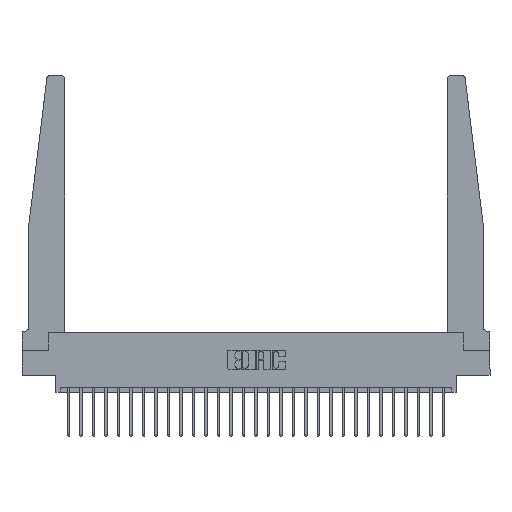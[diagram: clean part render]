
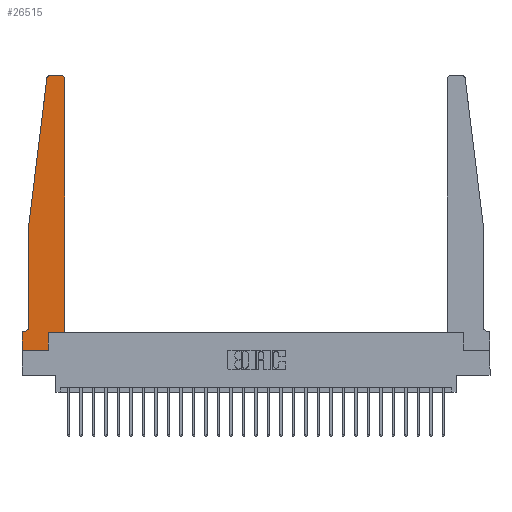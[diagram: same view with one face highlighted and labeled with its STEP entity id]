
A CAD part, top view. The second image highlights one B-rep face of the part: STEP entity #26515.
In plain terms, the highlighted planar face has unit normal (0, 0, 1).
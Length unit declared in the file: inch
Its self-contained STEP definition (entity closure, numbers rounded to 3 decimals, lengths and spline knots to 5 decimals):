
#359 = CARTESIAN_POINT ( 'NONE',  ( 0., 0., 0.37 ) ) ;
#526 = PLANE ( 'NONE',  #13266 ) ;
#586 = VERTEX_POINT ( 'NONE', #23461 ) ;
#639 = DIRECTION ( 'NONE',  ( -1., 0., 0. ) ) ;
#808 = DIRECTION ( 'NONE',  ( 1., 0., 0. ) ) ;
#1301 = LINE ( 'NONE', #24404, #22584 ) ;
#1389 = LINE ( 'NONE', #4986, #22674 ) ;
#1801 = VECTOR ( 'NONE', #2415, 39.37008 ) ;
#1988 = CARTESIAN_POINT ( 'NONE',  ( 0., 0., 0.37 ) ) ;
#2281 = CARTESIAN_POINT ( 'NONE',  ( 0.425, 0.18, 0.37 ) ) ;
#2287 = VECTOR ( 'NONE', #23270, 39.37008 ) ;
#2310 = VERTEX_POINT ( 'NONE', #2281 ) ;
#2415 = DIRECTION ( 'NONE',  ( -1., 0., 0. ) ) ;
#2443 = EDGE_CURVE ( 'NONE', #22834, #11309, #18690, .T. ) ;
#2521 = EDGE_CURVE ( 'NONE', #2310, #586, #22271, .T. ) ;
#2590 = DIRECTION ( 'NONE',  ( 0., 0., 1. ) ) ;
#2798 = EDGE_CURVE ( 'NONE', #4115, #15857, #1301, .T. ) ;
#3279 = CARTESIAN_POINT ( 'NONE',  ( 0.065, 1.25, 0.37 ) ) ;
#4115 = VERTEX_POINT ( 'NONE', #8124 ) ;
#4144 = VERTEX_POINT ( 'NONE', #16517 ) ;
#4646 = DIRECTION ( 'NONE',  ( 1., 0., 0. ) ) ;
#4750 = VECTOR ( 'NONE', #25264, 39.37008 ) ;
#4986 = CARTESIAN_POINT ( 'NONE',  ( 0.425, 0.18, 0.37 ) ) ;
#5061 = LINE ( 'NONE', #14219, #25661 ) ;
#5271 = CIRCLE ( 'NONE', #26112, 0.05 ) ;
#5754 = EDGE_CURVE ( 'NONE', #16105, #7443, #5061, .T. ) ;
#5853 = DIRECTION ( 'NONE',  ( -0.122, -0.992, 0. ) ) ;
#5947 = DIRECTION ( 'NONE',  ( -1., 0., 0. ) ) ;
#6760 = CARTESIAN_POINT ( 'NONE',  ( 0.2605, 0.18, 0.37 ) ) ;
#7409 = EDGE_CURVE ( 'NONE', #11993, #14815, #23071, .T. ) ;
#7443 = VERTEX_POINT ( 'NONE', #359 ) ;
#8124 = CARTESIAN_POINT ( 'NONE',  ( 0.24675, 2.72367, 0.37 ) ) ;
#9152 = EDGE_CURVE ( 'NONE', #20846, #4144, #5271, .T. ) ;
#11309 = VERTEX_POINT ( 'NONE', #25586 ) ;
#11506 = AXIS2_PLACEMENT_3D ( 'NONE', #14929, #2590, #17006 ) ;
#11908 = VECTOR ( 'NONE', #19368, 39.37008 ) ;
#11993 = VERTEX_POINT ( 'NONE', #21613 ) ;
#12822 = VECTOR ( 'NONE', #5947, 39.37008 ) ;
#12933 = DIRECTION ( 'NONE',  ( 0., 0., -1. ) ) ;
#13107 = DIRECTION ( 'NONE',  ( 0., 0., 1. ) ) ;
#13266 = AXIS2_PLACEMENT_3D ( 'NONE', #14891, #16970, #4646 ) ;
#14219 = CARTESIAN_POINT ( 'NONE',  ( 0., 0., 0.37 ) ) ;
#14815 = VERTEX_POINT ( 'NONE', #16593 ) ;
#14891 = CARTESIAN_POINT ( 'NONE',  ( 0., 0.1875, 0.37 ) ) ;
#14929 = CARTESIAN_POINT ( 'NONE',  ( 0.395, 2.72, 0.37 ) ) ;
#15441 = EDGE_LOOP ( 'NONE', ( #17378, #18001, #19680, #18299, #18963, #18697, #19303, #19280, #19360, #21789, #22783, #19728 ) ) ;
#15857 = VERTEX_POINT ( 'NONE', #3279 ) ;
#16017 = FACE_OUTER_BOUND ( 'NONE', #15441, .T. ) ;
#16105 = VERTEX_POINT ( 'NONE', #20054 ) ;
#16517 = CARTESIAN_POINT ( 'NONE',  ( 0.015, 0.1875, 0.37 ) ) ;
#16593 = CARTESIAN_POINT ( 'NONE',  ( 0.27653, 2.75, 0.37 ) ) ;
#16970 = DIRECTION ( 'NONE',  ( 0., 0., 1. ) ) ;
#17006 = DIRECTION ( 'NONE',  ( 1., 0., 0. ) ) ;
#17037 = VECTOR ( 'NONE', #22606, 39.37008 ) ;
#17378 = ORIENTED_EDGE ( 'NONE', *, *, #7409, .T. ) ;
#17654 = LINE ( 'NONE', #1988, #17037 ) ;
#17680 = AXIS2_PLACEMENT_3D ( 'NONE', #25440, #13107, #808 ) ;
#18001 = ORIENTED_EDGE ( 'NONE', *, *, #21928, .T. ) ;
#18299 = ORIENTED_EDGE ( 'NONE', *, *, #20100, .T. ) ;
#18690 = LINE ( 'NONE', #6760, #2287 ) ;
#18697 = ORIENTED_EDGE ( 'NONE', *, *, #19108, .T. ) ;
#18963 = ORIENTED_EDGE ( 'NONE', *, *, #9152, .T. ) ;
#19108 = EDGE_CURVE ( 'NONE', #4144, #16105, #23168, .T. ) ;
#19280 = ORIENTED_EDGE ( 'NONE', *, *, #25727, .T. ) ;
#19303 = ORIENTED_EDGE ( 'NONE', *, *, #5754, .T. ) ;
#19360 = ORIENTED_EDGE ( 'NONE', *, *, #2443, .T. ) ;
#19368 = DIRECTION ( 'NONE',  ( 0., 1., 0. ) ) ;
#19673 = CARTESIAN_POINT ( 'NONE',  ( 0.2605, 0., 0.37 ) ) ;
#19680 = ORIENTED_EDGE ( 'NONE', *, *, #2798, .T. ) ;
#19728 = ORIENTED_EDGE ( 'NONE', *, *, #25915, .T. ) ;
#19898 = CARTESIAN_POINT ( 'NONE',  ( 0.065, 0.2375, 0.37 ) ) ;
#20054 = CARTESIAN_POINT ( 'NONE',  ( 0., 0.1875, 0.37 ) ) ;
#20100 = EDGE_CURVE ( 'NONE', #15857, #20846, #26626, .T. ) ;
#20364 = CARTESIAN_POINT ( 'NONE',  ( 0.065, 0.1875, 0.37 ) ) ;
#20448 = DIRECTION ( 'NONE',  ( 0., -1., 0. ) ) ;
#20846 = VERTEX_POINT ( 'NONE', #19898 ) ;
#21069 = CIRCLE ( 'NONE', #17680, 0.03 ) ;
#21457 = CARTESIAN_POINT ( 'NONE',  ( 0.425, 0.18, 0.37 ) ) ;
#21613 = CARTESIAN_POINT ( 'NONE',  ( 0.395, 2.75, 0.37 ) ) ;
#21789 = ORIENTED_EDGE ( 'NONE', *, *, #22095, .T. ) ;
#21928 = EDGE_CURVE ( 'NONE', #14815, #4115, #21069, .T. ) ;
#22095 = EDGE_CURVE ( 'NONE', #11309, #2310, #1389, .T. ) ;
#22271 = LINE ( 'NONE', #21457, #11908 ) ;
#22584 = VECTOR ( 'NONE', #5853, 39.37008 ) ;
#22606 = DIRECTION ( 'NONE',  ( 1., 0., 0. ) ) ;
#22674 = VECTOR ( 'NONE', #25488, 39.37008 ) ;
#22783 = ORIENTED_EDGE ( 'NONE', *, *, #2521, .T. ) ;
#22834 = VERTEX_POINT ( 'NONE', #19673 ) ;
#23071 = LINE ( 'NONE', #24994, #1801 ) ;
#23168 = LINE ( 'NONE', #20364, #12822 ) ;
#23214 = CARTESIAN_POINT ( 'NONE',  ( 0.065, 1.25, 0.37 ) ) ;
#23270 = DIRECTION ( 'NONE',  ( 0., 1., 0. ) ) ;
#23461 = CARTESIAN_POINT ( 'NONE',  ( 0.425, 2.72, 0.37 ) ) ;
#23477 = CIRCLE ( 'NONE', #11506, 0.03 ) ;
#24404 = CARTESIAN_POINT ( 'NONE',  ( 0.065, 1.25, 0.37 ) ) ;
#24994 = CARTESIAN_POINT ( 'NONE',  ( 0.25, 2.75, 0.37 ) ) ;
#25264 = DIRECTION ( 'NONE',  ( 0., -1., 0. ) ) ;
#25270 = CARTESIAN_POINT ( 'NONE',  ( 0.015, 0.2375, 0.37 ) ) ;
#25440 = CARTESIAN_POINT ( 'NONE',  ( 0.27653, 2.72, 0.37 ) ) ;
#25488 = DIRECTION ( 'NONE',  ( 1., 0., 0. ) ) ;
#25586 = CARTESIAN_POINT ( 'NONE',  ( 0.2605, 0.18, 0.37 ) ) ;
#25661 = VECTOR ( 'NONE', #20448, 39.37008 ) ;
#25727 = EDGE_CURVE ( 'NONE', #7443, #22834, #17654, .T. ) ;
#25915 = EDGE_CURVE ( 'NONE', #586, #11993, #23477, .T. ) ;
#26112 = AXIS2_PLACEMENT_3D ( 'NONE', #25270, #12933, #639 ) ;
#26515 = ADVANCED_FACE ( 'NONE', ( #16017 ), #526, .T. ) ;
#26626 = LINE ( 'NONE', #23214, #4750 ) ;
